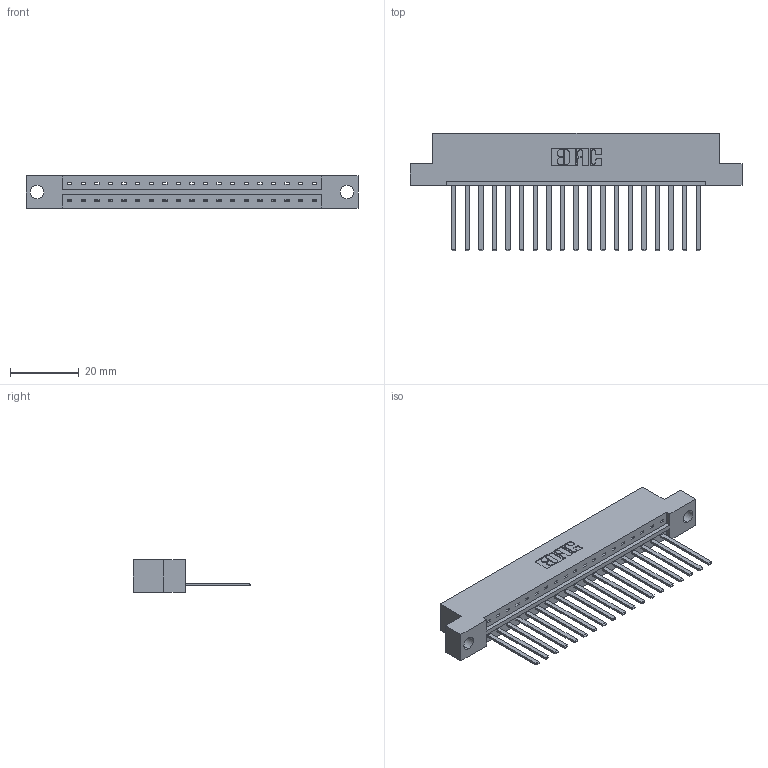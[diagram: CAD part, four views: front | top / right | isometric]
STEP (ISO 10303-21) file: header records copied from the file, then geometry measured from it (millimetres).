
FILE_DESCRIPTION (( 'STEP AP203' ), '1' );
FILE_NAME ('833-019-544-104.STEP', '2020-06-01T00:47:05', ( '' ), ( '' ), 'SwSTEP 2.0', 'SolidWorks 2020', '' );
FILE_SCHEMA (( 'CONFIG_CONTROL_DESIGN' ));
Length unit declared in the file: inch
Products named in the file (3): 833 Part_Flush - .156 Dia - TH; 345-292-001_345-293-144; 833-019-544-104
Assembly tree (20 placements, depth 2):
  833-019-544-104
    833 Part_Flush - .156 Dia - TH
    345-292-001_345-293-144  x19
Bounding box: 96.82 x 34.3 x 9.4 mm (x, y, z)
Volume: 9677.7 mm3; surface area: 10831.4 mm2
Topology: 20 solids, 20 shells, 1102 faces, 3313 edges, 2182 vertices
Faces by surface type: plane 792, cylinder 310
Entity records: 14409 total; most frequent: CARTESIAN_POINT 2495, ORIENTED_EDGE 2450, DIRECTION 2147, EDGE_CURVE 1225, LINE 1101, VECTOR 1101, VERTEX_POINT 814, AXIS2_PLACEMENT_3D 523
